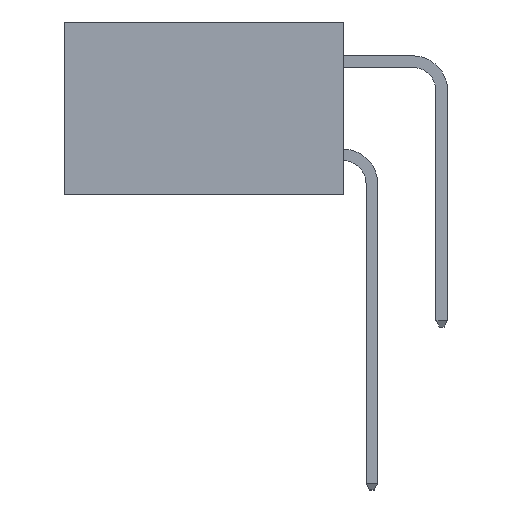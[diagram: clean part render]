
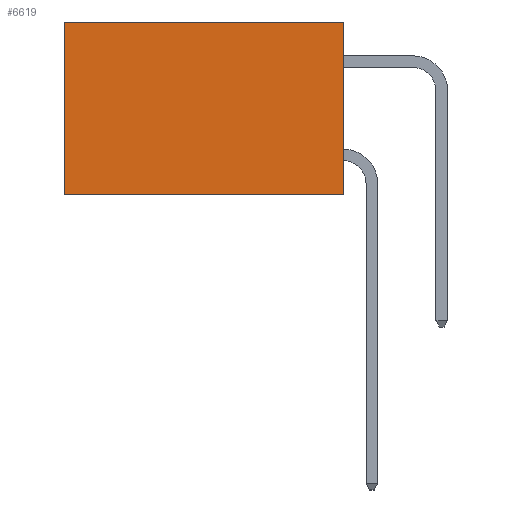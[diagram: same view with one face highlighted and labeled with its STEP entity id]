
A CAD part, left-side view. The second image highlights one B-rep face of the part: STEP entity #6619.
In plain terms, the highlighted planar face has unit normal (-1, 0, 0).
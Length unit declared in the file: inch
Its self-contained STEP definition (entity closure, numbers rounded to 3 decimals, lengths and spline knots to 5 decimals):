
#76 = CARTESIAN_POINT ( 'NONE',  ( 0.2615, 0.6, -0.37 ) ) ;
#183 = PLANE ( 'NONE',  #4010 ) ;
#2198 = LINE ( 'NONE', #7503, #12313 ) ;
#2262 = LINE ( 'NONE', #9295, #13219 ) ;
#3061 = CARTESIAN_POINT ( 'NONE',  ( 0.2615, 0., -0.37 ) ) ;
#3064 = CARTESIAN_POINT ( 'NONE',  ( 0.2615, 0.6, 0. ) ) ;
#3289 = VERTEX_POINT ( 'NONE', #4982 ) ;
#3455 = VERTEX_POINT ( 'NONE', #76 ) ;
#4010 = AXIS2_PLACEMENT_3D ( 'NONE', #8546, #13133, #13130 ) ;
#4110 = ORIENTED_EDGE ( 'NONE', *, *, #13395, .F. ) ;
#4982 = CARTESIAN_POINT ( 'NONE',  ( 0.2615, 0., 0. ) ) ;
#5061 = ORIENTED_EDGE ( 'NONE', *, *, #16353, .F. ) ;
#5321 = VERTEX_POINT ( 'NONE', #3061 ) ;
#5902 = LINE ( 'NONE', #15755, #12701 ) ;
#6281 = ORIENTED_EDGE ( 'NONE', *, *, #9162, .T. ) ;
#6619 = ADVANCED_FACE ( 'NONE', ( #14302 ), #183, .F. ) ;
#7370 = DIRECTION ( 'NONE',  ( 0., 1., 0. ) ) ;
#7472 = DIRECTION ( 'NONE',  ( 0., 0., -1. ) ) ;
#7503 = CARTESIAN_POINT ( 'NONE',  ( 0.2615, 0., 0. ) ) ;
#8546 = CARTESIAN_POINT ( 'NONE',  ( 0.2615, 0., -0.37 ) ) ;
#9162 = EDGE_CURVE ( 'NONE', #3289, #16212, #2198, .T. ) ;
#9295 = CARTESIAN_POINT ( 'NONE',  ( 0.2615, 0., -0.37 ) ) ;
#9500 = LINE ( 'NONE', #16913, #16243 ) ;
#10542 = EDGE_CURVE ( 'NONE', #16212, #3455, #5902, .T. ) ;
#12083 = EDGE_LOOP ( 'NONE', ( #17601, #4110, #5061, #6281 ) ) ;
#12313 = VECTOR ( 'NONE', #7370, 39.37008 ) ;
#12701 = VECTOR ( 'NONE', #15461, 39.37008 ) ;
#13130 = DIRECTION ( 'NONE',  ( 0., 0., -1. ) ) ;
#13133 = DIRECTION ( 'NONE',  ( 1., 0., 0. ) ) ;
#13219 = VECTOR ( 'NONE', #14688, 39.37008 ) ;
#13395 = EDGE_CURVE ( 'NONE', #5321, #3455, #2262, .T. ) ;
#14302 = FACE_OUTER_BOUND ( 'NONE', #12083, .T. ) ;
#14688 = DIRECTION ( 'NONE',  ( 0., 1., 0. ) ) ;
#15461 = DIRECTION ( 'NONE',  ( 0., 0., -1. ) ) ;
#15755 = CARTESIAN_POINT ( 'NONE',  ( 0.2615, 0.6, -0.37 ) ) ;
#16212 = VERTEX_POINT ( 'NONE', #3064 ) ;
#16243 = VECTOR ( 'NONE', #7472, 39.37008 ) ;
#16353 = EDGE_CURVE ( 'NONE', #3289, #5321, #9500, .T. ) ;
#16913 = CARTESIAN_POINT ( 'NONE',  ( 0.2615, 0., -0.37 ) ) ;
#17601 = ORIENTED_EDGE ( 'NONE', *, *, #10542, .T. ) ;
